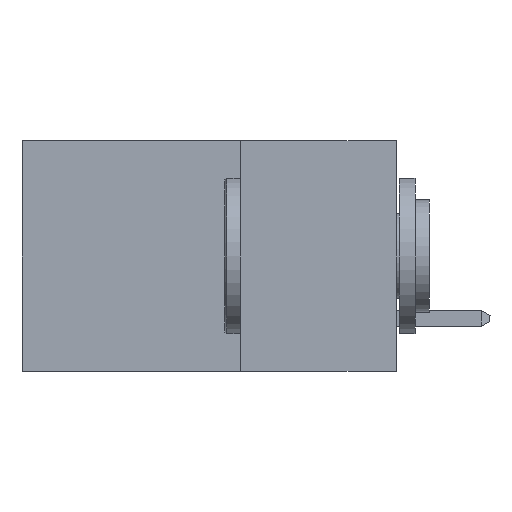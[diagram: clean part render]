
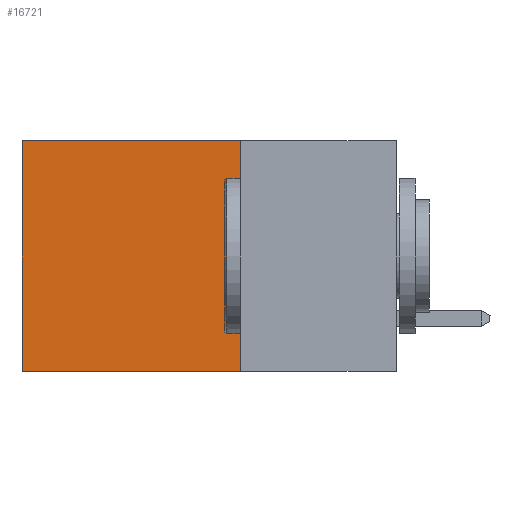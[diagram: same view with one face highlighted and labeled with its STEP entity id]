
A CAD part, left-side view. The second image highlights one B-rep face of the part: STEP entity #16721.
In plain terms, the highlighted planar face has unit normal (-1, 0, 0).
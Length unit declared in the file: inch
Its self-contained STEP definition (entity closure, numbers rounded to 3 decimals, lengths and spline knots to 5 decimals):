
#491 = VECTOR ( 'NONE', #18406, 39.37008 ) ;
#925 = DIRECTION ( 'NONE',  ( 1., 0., 0. ) ) ;
#1339 = EDGE_CURVE ( 'NONE', #22235, #15788, #20905, .T. ) ;
#1791 = VERTEX_POINT ( 'NONE', #2938 ) ;
#2407 = CARTESIAN_POINT ( 'NONE',  ( 0.2615, 0.25, 0. ) ) ;
#2938 = CARTESIAN_POINT ( 'NONE',  ( 0.2615, 0.6, -0.37 ) ) ;
#3421 = CARTESIAN_POINT ( 'NONE',  ( 0.2615, 0.25, -0.37 ) ) ;
#3827 = LINE ( 'NONE', #16381, #12670 ) ;
#5020 = CARTESIAN_POINT ( 'NONE',  ( 0.2615, 0.6, -0.37 ) ) ;
#6650 = VECTOR ( 'NONE', #13793, 39.37008 ) ;
#7872 = VECTOR ( 'NONE', #20562, 39.37008 ) ;
#8620 = VERTEX_POINT ( 'NONE', #17485 ) ;
#11650 = CARTESIAN_POINT ( 'NONE',  ( 0.2615, 0.25, -0.37 ) ) ;
#12064 = ORIENTED_EDGE ( 'NONE', *, *, #1339, .F. ) ;
#12544 = EDGE_LOOP ( 'NONE', ( #12802, #16815, #12064, #20594 ) ) ;
#12670 = VECTOR ( 'NONE', #18094, 39.37008 ) ;
#12802 = ORIENTED_EDGE ( 'NONE', *, *, #19542, .T. ) ;
#12917 = PLANE ( 'NONE',  #21970 ) ;
#13368 = DIRECTION ( 'NONE',  ( 0., 0., -1. ) ) ;
#13793 = DIRECTION ( 'NONE',  ( 0., 0., -1. ) ) ;
#14507 = EDGE_CURVE ( 'NONE', #22235, #8620, #14653, .T. ) ;
#14653 = LINE ( 'NONE', #20091, #491 ) ;
#15788 = VERTEX_POINT ( 'NONE', #3421 ) ;
#16048 = EDGE_CURVE ( 'NONE', #15788, #1791, #3827, .T. ) ;
#16381 = CARTESIAN_POINT ( 'NONE',  ( 0.2615, 0.25, -0.37 ) ) ;
#16721 = ADVANCED_FACE ( 'NONE', ( #20358 ), #12917, .F. ) ;
#16815 = ORIENTED_EDGE ( 'NONE', *, *, #16048, .F. ) ;
#17485 = CARTESIAN_POINT ( 'NONE',  ( 0.2615, 0.6, 0. ) ) ;
#18094 = DIRECTION ( 'NONE',  ( 0., 1., 0. ) ) ;
#18406 = DIRECTION ( 'NONE',  ( 0., 1., 0. ) ) ;
#19542 = EDGE_CURVE ( 'NONE', #8620, #1791, #20324, .T. ) ;
#20091 = CARTESIAN_POINT ( 'NONE',  ( 0.2615, 0.25, 0. ) ) ;
#20324 = LINE ( 'NONE', #5020, #6650 ) ;
#20358 = FACE_OUTER_BOUND ( 'NONE', #12544, .T. ) ;
#20562 = DIRECTION ( 'NONE',  ( 0., 0., -1. ) ) ;
#20594 = ORIENTED_EDGE ( 'NONE', *, *, #14507, .T. ) ;
#20905 = LINE ( 'NONE', #20944, #7872 ) ;
#20944 = CARTESIAN_POINT ( 'NONE',  ( 0.2615, 0.25, -0.37 ) ) ;
#21970 = AXIS2_PLACEMENT_3D ( 'NONE', #11650, #925, #13368 ) ;
#22235 = VERTEX_POINT ( 'NONE', #2407 ) ;
